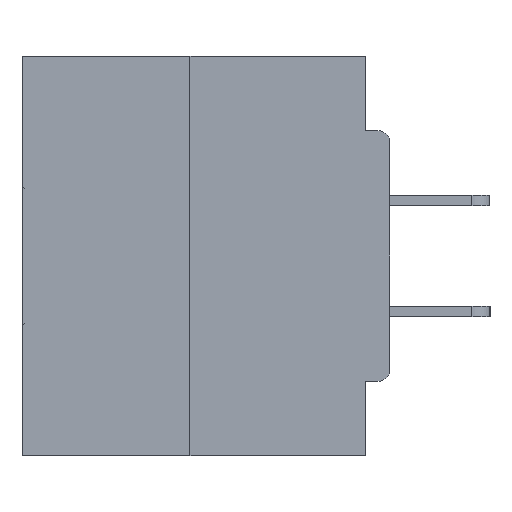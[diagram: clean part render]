
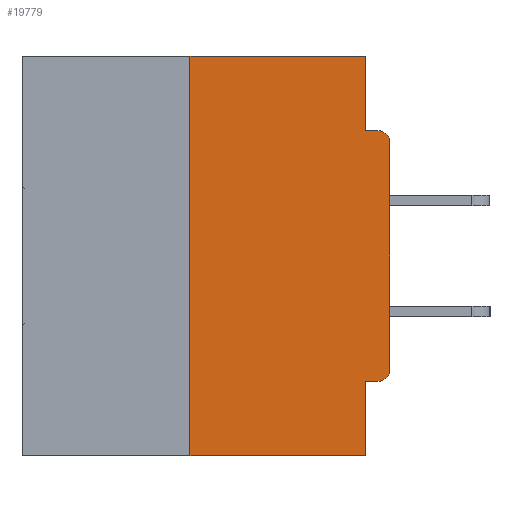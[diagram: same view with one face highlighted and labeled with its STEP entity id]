
A CAD part, left-side view. The second image highlights one B-rep face of the part: STEP entity #19779.
In plain terms, the highlighted planar face has unit normal (-1, 0, 0).
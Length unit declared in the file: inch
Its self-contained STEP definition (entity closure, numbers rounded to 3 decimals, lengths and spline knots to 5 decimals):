
#159 = DIRECTION ( 'NONE',  ( 0., -1., 0. ) ) ;
#365 = CIRCLE ( 'NONE', #11029, 0.015 ) ;
#529 = CARTESIAN_POINT ( 'NONE',  ( 0., 0.015, -0.1085 ) ) ;
#1155 = DIRECTION ( 'NONE',  ( -1., 0., 0. ) ) ;
#1699 = CARTESIAN_POINT ( 'NONE',  ( 0., 0.031, -0.0935 ) ) ;
#2190 = AXIS2_PLACEMENT_3D ( 'NONE', #529, #1155, #10518 ) ;
#2532 = EDGE_CURVE ( 'NONE', #17585, #10424, #9438, .T. ) ;
#2589 = CARTESIAN_POINT ( 'NONE',  ( 0., 0.031, -0.5 ) ) ;
#2616 = LINE ( 'NONE', #36650, #3400 ) ;
#3274 = VERTEX_POINT ( 'NONE', #36885 ) ;
#3400 = VECTOR ( 'NONE', #30603, 39.37008 ) ;
#4254 = DIRECTION ( 'NONE',  ( 0., -1., 0. ) ) ;
#5330 = CARTESIAN_POINT ( 'NONE',  ( 0., 0., -0.1085 ) ) ;
#6214 = VERTEX_POINT ( 'NONE', #22529 ) ;
#7866 = EDGE_LOOP ( 'NONE', ( #26047, #22649, #23103, #10329, #29435, #17767, #12318, #32237, #33259, #17196 ) ) ;
#8027 = CARTESIAN_POINT ( 'NONE',  ( 0., 0.015, -0.3915 ) ) ;
#8416 = EDGE_CURVE ( 'NONE', #10424, #25101, #27303, .T. ) ;
#8477 = FACE_OUTER_BOUND ( 'NONE', #7866, .T. ) ;
#9351 = DIRECTION ( 'NONE',  ( 0., 1., 0. ) ) ;
#9438 = LINE ( 'NONE', #40530, #23038 ) ;
#10156 = EDGE_CURVE ( 'NONE', #6214, #3274, #365, .T. ) ;
#10228 = VERTEX_POINT ( 'NONE', #2589 ) ;
#10329 = ORIENTED_EDGE ( 'NONE', *, *, #40091, .F. ) ;
#10424 = VERTEX_POINT ( 'NONE', #23231 ) ;
#10518 = DIRECTION ( 'NONE',  ( 0., 0., -1. ) ) ;
#10779 = DIRECTION ( 'NONE',  ( 0., 0., 1. ) ) ;
#11029 = AXIS2_PLACEMENT_3D ( 'NONE', #8027, #11344, #21266 ) ;
#11344 = DIRECTION ( 'NONE',  ( -1., 0., 0. ) ) ;
#11799 = CARTESIAN_POINT ( 'NONE',  ( 0., 0.031, 0. ) ) ;
#12137 = EDGE_CURVE ( 'NONE', #6214, #39177, #12457, .T. ) ;
#12318 = ORIENTED_EDGE ( 'NONE', *, *, #20921, .T. ) ;
#12457 = LINE ( 'NONE', #25663, #25861 ) ;
#12847 = VERTEX_POINT ( 'NONE', #35156 ) ;
#15030 = VERTEX_POINT ( 'NONE', #5330 ) ;
#16834 = CIRCLE ( 'NONE', #2190, 0.015 ) ;
#17196 = ORIENTED_EDGE ( 'NONE', *, *, #40979, .F. ) ;
#17388 = DIRECTION ( 'NONE',  ( 0., -1., 0. ) ) ;
#17390 = CARTESIAN_POINT ( 'NONE',  ( 0., 0., 0. ) ) ;
#17585 = VERTEX_POINT ( 'NONE', #28487 ) ;
#17767 = ORIENTED_EDGE ( 'NONE', *, *, #10156, .T. ) ;
#18013 = CARTESIAN_POINT ( 'NONE',  ( 0., 0.46, 0. ) ) ;
#19669 = LINE ( 'NONE', #26055, #35254 ) ;
#19779 = ADVANCED_FACE ( 'NONE', ( #8477 ), #24799, .F. ) ;
#20921 = EDGE_CURVE ( 'NONE', #3274, #15030, #30217, .T. ) ;
#21266 = DIRECTION ( 'NONE',  ( 0., 0., -1. ) ) ;
#21505 = CARTESIAN_POINT ( 'NONE',  ( 0., 0.46, 0. ) ) ;
#22529 = CARTESIAN_POINT ( 'NONE',  ( 0., 0.015, -0.4065 ) ) ;
#22649 = ORIENTED_EDGE ( 'NONE', *, *, #2532, .F. ) ;
#22675 = LINE ( 'NONE', #32615, #34476 ) ;
#22717 = CARTESIAN_POINT ( 'NONE',  ( 0., 0.031, 0. ) ) ;
#23038 = VECTOR ( 'NONE', #34694, 39.37008 ) ;
#23103 = ORIENTED_EDGE ( 'NONE', *, *, #27209, .T. ) ;
#23231 = CARTESIAN_POINT ( 'NONE',  ( 0., 0.25, 0. ) ) ;
#23722 = EDGE_CURVE ( 'NONE', #26154, #12847, #19669, .T. ) ;
#24220 = DIRECTION ( 'NONE',  ( 0., 0., -1. ) ) ;
#24414 = LINE ( 'NONE', #11799, #24633 ) ;
#24633 = VECTOR ( 'NONE', #24220, 39.37008 ) ;
#24799 = PLANE ( 'NONE',  #27437 ) ;
#24986 = DIRECTION ( 'NONE',  ( 1., 0., 0. ) ) ;
#25101 = VERTEX_POINT ( 'NONE', #22717 ) ;
#25663 = CARTESIAN_POINT ( 'NONE',  ( 0., 0., -0.4065 ) ) ;
#25861 = VECTOR ( 'NONE', #9351, 39.37008 ) ;
#26047 = ORIENTED_EDGE ( 'NONE', *, *, #8416, .F. ) ;
#26055 = CARTESIAN_POINT ( 'NONE',  ( 0., 0., -0.0935 ) ) ;
#26154 = VERTEX_POINT ( 'NONE', #1699 ) ;
#26965 = VECTOR ( 'NONE', #17388, 39.37008 ) ;
#27209 = EDGE_CURVE ( 'NONE', #17585, #10228, #22675, .T. ) ;
#27303 = LINE ( 'NONE', #21505, #26965 ) ;
#27437 = AXIS2_PLACEMENT_3D ( 'NONE', #18013, #24986, #37658 ) ;
#28487 = CARTESIAN_POINT ( 'NONE',  ( 0., 0.25, -0.5 ) ) ;
#29435 = ORIENTED_EDGE ( 'NONE', *, *, #12137, .F. ) ;
#30217 = LINE ( 'NONE', #17390, #31163 ) ;
#30603 = DIRECTION ( 'NONE',  ( 0., 0., -1. ) ) ;
#30717 = EDGE_CURVE ( 'NONE', #15030, #12847, #16834, .T. ) ;
#31163 = VECTOR ( 'NONE', #10779, 39.37008 ) ;
#32237 = ORIENTED_EDGE ( 'NONE', *, *, #30717, .T. ) ;
#32615 = CARTESIAN_POINT ( 'NONE',  ( 0., 0.46, -0.5 ) ) ;
#33259 = ORIENTED_EDGE ( 'NONE', *, *, #23722, .F. ) ;
#34476 = VECTOR ( 'NONE', #4254, 39.37008 ) ;
#34694 = DIRECTION ( 'NONE',  ( 0., 0., 1. ) ) ;
#35156 = CARTESIAN_POINT ( 'NONE',  ( 0., 0.015, -0.0935 ) ) ;
#35254 = VECTOR ( 'NONE', #159, 39.37008 ) ;
#36650 = CARTESIAN_POINT ( 'NONE',  ( 0., 0.031, -0.5 ) ) ;
#36885 = CARTESIAN_POINT ( 'NONE',  ( 0., 0., -0.3915 ) ) ;
#37658 = DIRECTION ( 'NONE',  ( 0., 0., -1. ) ) ;
#39177 = VERTEX_POINT ( 'NONE', #40263 ) ;
#40091 = EDGE_CURVE ( 'NONE', #39177, #10228, #2616, .T. ) ;
#40263 = CARTESIAN_POINT ( 'NONE',  ( 0., 0.031, -0.4065 ) ) ;
#40530 = CARTESIAN_POINT ( 'NONE',  ( 0., 0.25, 0. ) ) ;
#40979 = EDGE_CURVE ( 'NONE', #25101, #26154, #24414, .T. ) ;
